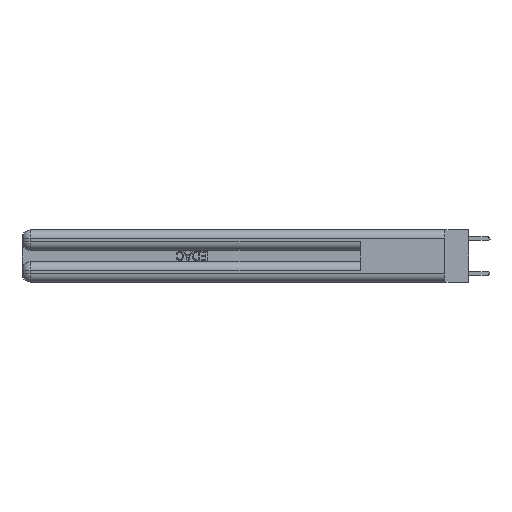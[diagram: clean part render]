
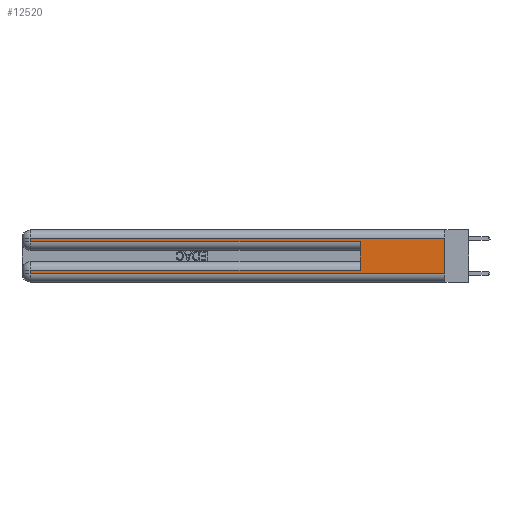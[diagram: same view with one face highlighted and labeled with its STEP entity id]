
A CAD part, left-side view. The second image highlights one B-rep face of the part: STEP entity #12520.
In plain terms, the highlighted planar face has unit normal (-1, 0, 0).
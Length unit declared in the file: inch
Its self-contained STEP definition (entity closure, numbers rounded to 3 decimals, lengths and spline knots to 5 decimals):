
#585 = LINE ( 'NONE', #24576, #20887 ) ;
#621 = AXIS2_PLACEMENT_3D ( 'NONE', #27388, #2107, #19894 ) ;
#1434 = DIRECTION ( 'NONE',  ( 0., 0., -1. ) ) ;
#1663 = ORIENTED_EDGE ( 'NONE', *, *, #25678, .T. ) ;
#2085 = VECTOR ( 'NONE', #26558, 39.37008 ) ;
#2107 = DIRECTION ( 'NONE',  ( 1., 0., 0. ) ) ;
#2276 = EDGE_CURVE ( 'NONE', #16603, #7604, #32243, .T. ) ;
#3496 = DIRECTION ( 'NONE',  ( 0., 0., -1. ) ) ;
#4307 = CARTESIAN_POINT ( 'NONE',  ( 0., 0.6, 0.085 ) ) ;
#4955 = VERTEX_POINT ( 'NONE', #7388 ) ;
#5467 = FACE_OUTER_BOUND ( 'NONE', #20679, .T. ) ;
#5513 = ORIENTED_EDGE ( 'NONE', *, *, #2276, .T. ) ;
#5899 = CARTESIAN_POINT ( 'NONE',  ( 0., 0., 0.31 ) ) ;
#6321 = CARTESIAN_POINT ( 'NONE',  ( 0., 2.94, 0.37 ) ) ;
#7376 = VECTOR ( 'NONE', #23689, 39.37008 ) ;
#7388 = CARTESIAN_POINT ( 'NONE',  ( 0., 2.94, 0.285 ) ) ;
#7604 = VERTEX_POINT ( 'NONE', #15436 ) ;
#7730 = LINE ( 'NONE', #21140, #7376 ) ;
#8082 = CARTESIAN_POINT ( 'NONE',  ( 0., 2.94, 0.085 ) ) ;
#9036 = VECTOR ( 'NONE', #30252, 39.37008 ) ;
#9421 = DIRECTION ( 'NONE',  ( 0., 1., 0. ) ) ;
#9433 = CARTESIAN_POINT ( 'NONE',  ( 0., 0., 0.06 ) ) ;
#9537 = DIRECTION ( 'NONE',  ( 0., -1., 0. ) ) ;
#10577 = VECTOR ( 'NONE', #1434, 39.37008 ) ;
#10766 = VERTEX_POINT ( 'NONE', #15691 ) ;
#12482 = ORIENTED_EDGE ( 'NONE', *, *, #23747, .F. ) ;
#12520 = ADVANCED_FACE ( 'NONE', ( #5467 ), #17364, .F. ) ;
#12620 = EDGE_CURVE ( 'NONE', #4955, #10766, #17389, .T. ) ;
#13133 = EDGE_CURVE ( 'NONE', #20564, #16603, #585, .T. ) ;
#13611 = VERTEX_POINT ( 'NONE', #28846 ) ;
#14279 = ORIENTED_EDGE ( 'NONE', *, *, #32748, .T. ) ;
#15436 = CARTESIAN_POINT ( 'NONE',  ( 0., 2.94, 0.06 ) ) ;
#15501 = ORIENTED_EDGE ( 'NONE', *, *, #29854, .T. ) ;
#15650 = LINE ( 'NONE', #6321, #2085 ) ;
#15691 = CARTESIAN_POINT ( 'NONE',  ( 0., 0.6, 0.285 ) ) ;
#16248 = LINE ( 'NONE', #9433, #28892 ) ;
#16603 = VERTEX_POINT ( 'NONE', #8082 ) ;
#17364 = PLANE ( 'NONE',  #621 ) ;
#17389 = LINE ( 'NONE', #20114, #9036 ) ;
#19010 = CARTESIAN_POINT ( 'NONE',  ( 0., 2.94, 0.31 ) ) ;
#19651 = LINE ( 'NONE', #26176, #32229 ) ;
#19894 = DIRECTION ( 'NONE',  ( 0., 0., -1. ) ) ;
#20114 = CARTESIAN_POINT ( 'NONE',  ( 0., 0., 0.285 ) ) ;
#20564 = VERTEX_POINT ( 'NONE', #4307 ) ;
#20679 = EDGE_LOOP ( 'NONE', ( #12482, #14279, #15501, #22892, #20868, #21386, #5513, #1663 ) ) ;
#20768 = CARTESIAN_POINT ( 'NONE',  ( 0., 0., 0.06 ) ) ;
#20868 = ORIENTED_EDGE ( 'NONE', *, *, #28429, .F. ) ;
#20887 = VECTOR ( 'NONE', #9421, 39.37008 ) ;
#21140 = CARTESIAN_POINT ( 'NONE',  ( 0., 0.6, 0.145 ) ) ;
#21191 = DIRECTION ( 'NONE',  ( 0., 1., 0. ) ) ;
#21386 = ORIENTED_EDGE ( 'NONE', *, *, #13133, .T. ) ;
#22892 = ORIENTED_EDGE ( 'NONE', *, *, #12620, .T. ) ;
#23689 = DIRECTION ( 'NONE',  ( 0., 0., 1. ) ) ;
#23747 = EDGE_CURVE ( 'NONE', #13611, #30692, #19651, .T. ) ;
#23858 = VERTEX_POINT ( 'NONE', #19010 ) ;
#24576 = CARTESIAN_POINT ( 'NONE',  ( 0., 0., 0.085 ) ) ;
#25678 = EDGE_CURVE ( 'NONE', #7604, #30692, #16248, .T. ) ;
#26176 = CARTESIAN_POINT ( 'NONE',  ( 0., 0., 0.37 ) ) ;
#26558 = DIRECTION ( 'NONE',  ( 0., 0., -1. ) ) ;
#27140 = VECTOR ( 'NONE', #21191, 39.37008 ) ;
#27388 = CARTESIAN_POINT ( 'NONE',  ( 0., 0., 0.37 ) ) ;
#28280 = LINE ( 'NONE', #5899, #27140 ) ;
#28429 = EDGE_CURVE ( 'NONE', #20564, #10766, #7730, .T. ) ;
#28846 = CARTESIAN_POINT ( 'NONE',  ( 0., 0., 0.31 ) ) ;
#28892 = VECTOR ( 'NONE', #9537, 39.37008 ) ;
#29854 = EDGE_CURVE ( 'NONE', #23858, #4955, #15650, .T. ) ;
#30252 = DIRECTION ( 'NONE',  ( 0., -1., 0. ) ) ;
#30692 = VERTEX_POINT ( 'NONE', #20768 ) ;
#31755 = CARTESIAN_POINT ( 'NONE',  ( 0., 2.94, 0.37 ) ) ;
#32229 = VECTOR ( 'NONE', #3496, 39.37008 ) ;
#32243 = LINE ( 'NONE', #31755, #10577 ) ;
#32748 = EDGE_CURVE ( 'NONE', #13611, #23858, #28280, .T. ) ;
